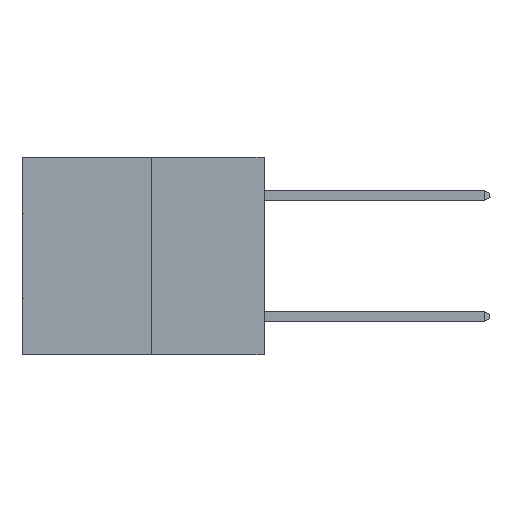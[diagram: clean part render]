
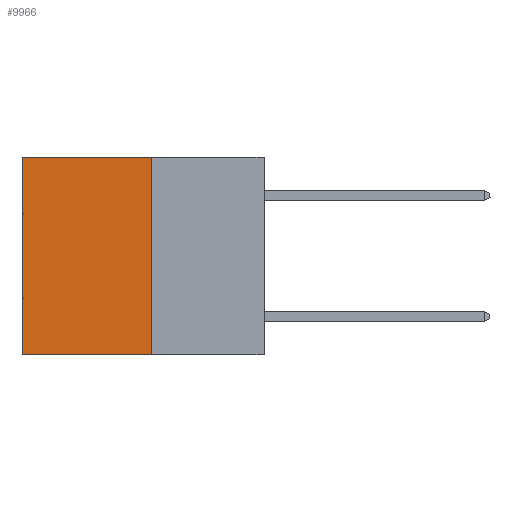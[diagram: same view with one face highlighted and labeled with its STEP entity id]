
A CAD part, left-side view. The second image highlights one B-rep face of the part: STEP entity #9966.
In plain terms, the highlighted planar face has unit normal (-1, 0, 0).
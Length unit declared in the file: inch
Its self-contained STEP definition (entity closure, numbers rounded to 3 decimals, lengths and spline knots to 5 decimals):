
#4025 = EDGE_CURVE ( 'NONE', #22567, #4618, #18072, .T. ) ;
#4471 = EDGE_CURVE ( 'NONE', #22567, #16719, #16841, .T. ) ;
#4618 = VERTEX_POINT ( 'NONE', #12587 ) ;
#5545 = DIRECTION ( 'NONE',  ( 0., 0., -1. ) ) ;
#5918 = DIRECTION ( 'NONE',  ( 0., 1., 0. ) ) ;
#6191 = ORIENTED_EDGE ( 'NONE', *, *, #4025, .T. ) ;
#7786 = CARTESIAN_POINT ( 'NONE',  ( 0.3165, 0.28, -0.49 ) ) ;
#8479 = ORIENTED_EDGE ( 'NONE', *, *, #13410, .F. ) ;
#9041 = CARTESIAN_POINT ( 'NONE',  ( 0.3165, 0.28, 0. ) ) ;
#9124 = CARTESIAN_POINT ( 'NONE',  ( 0.3165, 0.28, -0.49 ) ) ;
#9151 = AXIS2_PLACEMENT_3D ( 'NONE', #9124, #22027, #24582 ) ;
#9245 = CARTESIAN_POINT ( 'NONE',  ( 0.3165, 0.28, 0. ) ) ;
#9674 = ORIENTED_EDGE ( 'NONE', *, *, #4471, .F. ) ;
#9966 = ADVANCED_FACE ( 'NONE', ( #21328 ), #19512, .F. ) ;
#11243 = CARTESIAN_POINT ( 'NONE',  ( 0.3165, 0.28, -0.49 ) ) ;
#12587 = CARTESIAN_POINT ( 'NONE',  ( 0.3165, 0.6, 0. ) ) ;
#12809 = VERTEX_POINT ( 'NONE', #15880 ) ;
#13410 = EDGE_CURVE ( 'NONE', #16719, #12809, #18534, .T. ) ;
#14548 = VECTOR ( 'NONE', #5918, 39.37008 ) ;
#15880 = CARTESIAN_POINT ( 'NONE',  ( 0.3165, 0.6, -0.49 ) ) ;
#16719 = VERTEX_POINT ( 'NONE', #29215 ) ;
#16841 = LINE ( 'NONE', #7786, #24353 ) ;
#16866 = VECTOR ( 'NONE', #21405, 39.37008 ) ;
#17703 = LINE ( 'NONE', #25847, #31523 ) ;
#18072 = LINE ( 'NONE', #9041, #16866 ) ;
#18534 = LINE ( 'NONE', #11243, #14548 ) ;
#19512 = PLANE ( 'NONE',  #9151 ) ;
#20568 = EDGE_CURVE ( 'NONE', #4618, #12809, #17703, .T. ) ;
#21328 = FACE_OUTER_BOUND ( 'NONE', #32628, .T. ) ;
#21405 = DIRECTION ( 'NONE',  ( 0., 1., 0. ) ) ;
#22027 = DIRECTION ( 'NONE',  ( 1., 0., 0. ) ) ;
#22567 = VERTEX_POINT ( 'NONE', #9245 ) ;
#24353 = VECTOR ( 'NONE', #27988, 39.37008 ) ;
#24582 = DIRECTION ( 'NONE',  ( 0., 0., -1. ) ) ;
#25847 = CARTESIAN_POINT ( 'NONE',  ( 0.3165, 0.6, -0.49 ) ) ;
#27988 = DIRECTION ( 'NONE',  ( 0., 0., -1. ) ) ;
#29215 = CARTESIAN_POINT ( 'NONE',  ( 0.3165, 0.28, -0.49 ) ) ;
#30195 = ORIENTED_EDGE ( 'NONE', *, *, #20568, .T. ) ;
#31523 = VECTOR ( 'NONE', #5545, 39.37008 ) ;
#32628 = EDGE_LOOP ( 'NONE', ( #30195, #8479, #9674, #6191 ) ) ;
